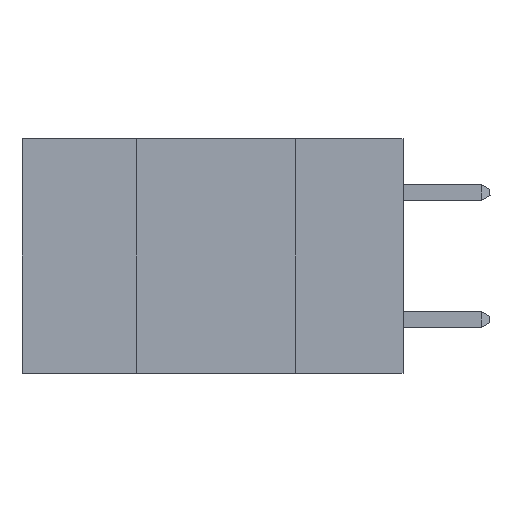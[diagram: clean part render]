
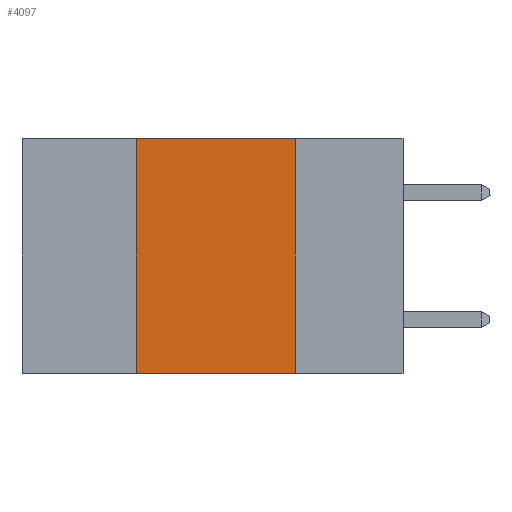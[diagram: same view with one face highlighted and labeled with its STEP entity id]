
A CAD part, left-side view. The second image highlights one B-rep face of the part: STEP entity #4097.
In plain terms, the highlighted planar face has unit normal (-1, 0, 0).
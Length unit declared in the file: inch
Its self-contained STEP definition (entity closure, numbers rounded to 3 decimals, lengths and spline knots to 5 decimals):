
#31 = ORIENTED_EDGE ( 'NONE', *, *, #10862, .F. ) ;
#633 = VERTEX_POINT ( 'NONE', #39062 ) ;
#1762 = CARTESIAN_POINT ( 'NONE',  ( 0., 0.6, 0. ) ) ;
#4097 = ADVANCED_FACE ( 'NONE', ( #11502 ), #10921, .F. ) ;
#6174 = VERTEX_POINT ( 'NONE', #28161 ) ;
#6518 = ORIENTED_EDGE ( 'NONE', *, *, #27044, .F. ) ;
#7352 = VECTOR ( 'NONE', #20428, 39.37008 ) ;
#8665 = DIRECTION ( 'NONE',  ( 0., 0., -1. ) ) ;
#8745 = DIRECTION ( 'NONE',  ( 0., 0., 1. ) ) ;
#10862 = EDGE_CURVE ( 'NONE', #25796, #633, #26006, .T. ) ;
#10921 = PLANE ( 'NONE',  #39763 ) ;
#11502 = FACE_OUTER_BOUND ( 'NONE', #34367, .T. ) ;
#12239 = VECTOR ( 'NONE', #17461, 39.37008 ) ;
#14487 = CARTESIAN_POINT ( 'NONE',  ( 0., 0.42, 0. ) ) ;
#14738 = VERTEX_POINT ( 'NONE', #14487 ) ;
#15838 = VECTOR ( 'NONE', #8745, 39.37008 ) ;
#17461 = DIRECTION ( 'NONE',  ( 0., 0., -1. ) ) ;
#20428 = DIRECTION ( 'NONE',  ( 0., -1., 0. ) ) ;
#20679 = LINE ( 'NONE', #33044, #27903 ) ;
#22603 = ORIENTED_EDGE ( 'NONE', *, *, #28092, .F. ) ;
#23889 = CARTESIAN_POINT ( 'NONE',  ( 0., 0.6, 0. ) ) ;
#24092 = DIRECTION ( 'NONE',  ( 1., 0., 0. ) ) ;
#25796 = VERTEX_POINT ( 'NONE', #32375 ) ;
#26006 = LINE ( 'NONE', #35311, #12239 ) ;
#27044 = EDGE_CURVE ( 'NONE', #14738, #25796, #29553, .T. ) ;
#27617 = CARTESIAN_POINT ( 'NONE',  ( 0., 0.42, 0. ) ) ;
#27903 = VECTOR ( 'NONE', #39920, 39.37008 ) ;
#28092 = EDGE_CURVE ( 'NONE', #6174, #14738, #36521, .T. ) ;
#28161 = CARTESIAN_POINT ( 'NONE',  ( 0., 0.42, -0.37 ) ) ;
#29553 = LINE ( 'NONE', #1762, #7352 ) ;
#32375 = CARTESIAN_POINT ( 'NONE',  ( 0., 0.17, 0. ) ) ;
#33044 = CARTESIAN_POINT ( 'NONE',  ( 0., 0.6, -0.37 ) ) ;
#34367 = EDGE_LOOP ( 'NONE', ( #31, #6518, #22603, #35448 ) ) ;
#35311 = CARTESIAN_POINT ( 'NONE',  ( 0., 0.17, 0. ) ) ;
#35448 = ORIENTED_EDGE ( 'NONE', *, *, #39099, .T. ) ;
#36521 = LINE ( 'NONE', #27617, #15838 ) ;
#39062 = CARTESIAN_POINT ( 'NONE',  ( 0., 0.17, -0.37 ) ) ;
#39099 = EDGE_CURVE ( 'NONE', #6174, #633, #20679, .T. ) ;
#39763 = AXIS2_PLACEMENT_3D ( 'NONE', #23889, #24092, #8665 ) ;
#39920 = DIRECTION ( 'NONE',  ( 0., -1., 0. ) ) ;
